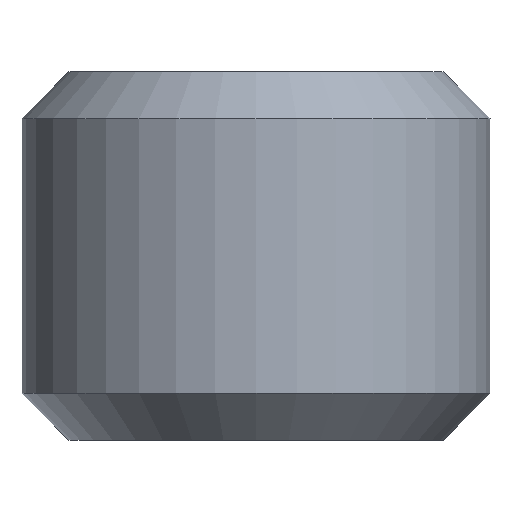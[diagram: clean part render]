
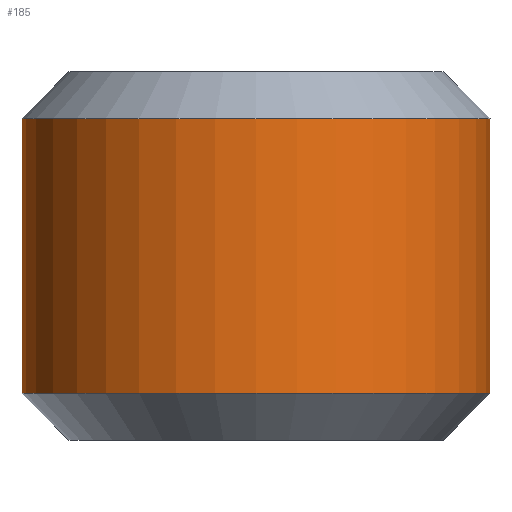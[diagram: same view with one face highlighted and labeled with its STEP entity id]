
A CAD part, left-side view. The second image highlights one B-rep face of the part: STEP entity #185.
In plain terms, the highlighted cylindrical face has radius 6.35 mm (diameter 12.7 mm), a partial arc.
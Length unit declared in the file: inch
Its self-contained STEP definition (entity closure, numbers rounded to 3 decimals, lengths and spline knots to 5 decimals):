
#6 = EDGE_CURVE ( 'NONE', #158, #228, #101, .T. ) ;
#10 = CARTESIAN_POINT ( 'NONE',  ( 0., -0.05315, 0.14685 ) ) ;
#11 = CARTESIAN_POINT ( 'NONE',  ( 0., -0.05315, 0.19685 ) ) ;
#32 = CARTESIAN_POINT ( 'NONE',  ( 0., -0.05315, -0.14685 ) ) ;
#34 = DIRECTION ( 'NONE',  ( 0., 0., -1. ) ) ;
#40 = ORIENTED_EDGE ( 'NONE', *, *, #6, .T. ) ;
#53 = ORIENTED_EDGE ( 'NONE', *, *, #182, .T. ) ;
#57 = VERTEX_POINT ( 'NONE', #237 ) ;
#78 = CARTESIAN_POINT ( 'NONE',  ( 0., 0.19685, -0.14685 ) ) ;
#99 = AXIS2_PLACEMENT_3D ( 'NONE', #134, #107, #240 ) ;
#101 = CIRCLE ( 'NONE', #143, 0.25 ) ;
#107 = DIRECTION ( 'NONE',  ( 0., 0., -1. ) ) ;
#109 = DIRECTION ( 'NONE',  ( 0., 0., -1. ) ) ;
#112 = ORIENTED_EDGE ( 'NONE', *, *, #178, .T. ) ;
#116 = AXIS2_PLACEMENT_3D ( 'NONE', #136, #109, #145 ) ;
#134 = CARTESIAN_POINT ( 'NONE',  ( 0., 0.19685, 0.19685 ) ) ;
#136 = CARTESIAN_POINT ( 'NONE',  ( 0., 0.19685, 0.14685 ) ) ;
#138 = CARTESIAN_POINT ( 'NONE',  ( 0., 0.44685, -0.14685 ) ) ;
#142 = ORIENTED_EDGE ( 'NONE', *, *, #192, .F. ) ;
#143 = AXIS2_PLACEMENT_3D ( 'NONE', #78, #154, #221 ) ;
#145 = DIRECTION ( 'NONE',  ( 0., -1., 0. ) ) ;
#148 = VECTOR ( 'NONE', #34, 39.37008 ) ;
#151 = LINE ( 'NONE', #11, #148 ) ;
#154 = DIRECTION ( 'NONE',  ( 0., 0., 1. ) ) ;
#158 = VERTEX_POINT ( 'NONE', #138 ) ;
#171 = CIRCLE ( 'NONE', #116, 0.25 ) ;
#178 = EDGE_CURVE ( 'NONE', #57, #158, #203, .T. ) ;
#180 = CYLINDRICAL_SURFACE ( 'NONE', #99, 0.25 ) ;
#182 = EDGE_CURVE ( 'NONE', #213, #57, #171, .T. ) ;
#185 = ADVANCED_FACE ( 'NONE', ( #193 ), #180, .T. ) ;
#192 = EDGE_CURVE ( 'NONE', #213, #228, #151, .T. ) ;
#193 = FACE_OUTER_BOUND ( 'NONE', #245, .T. ) ;
#200 = CARTESIAN_POINT ( 'NONE',  ( 0., 0.44685, 0.19685 ) ) ;
#203 = LINE ( 'NONE', #200, #225 ) ;
#213 = VERTEX_POINT ( 'NONE', #10 ) ;
#221 = DIRECTION ( 'NONE',  ( 0., -1., 0. ) ) ;
#225 = VECTOR ( 'NONE', #248, 39.37008 ) ;
#228 = VERTEX_POINT ( 'NONE', #32 ) ;
#237 = CARTESIAN_POINT ( 'NONE',  ( 0., 0.44685, 0.14685 ) ) ;
#240 = DIRECTION ( 'NONE',  ( 0., 1., 0. ) ) ;
#245 = EDGE_LOOP ( 'NONE', ( #142, #53, #112, #40 ) ) ;
#248 = DIRECTION ( 'NONE',  ( 0., 0., -1. ) ) ;
